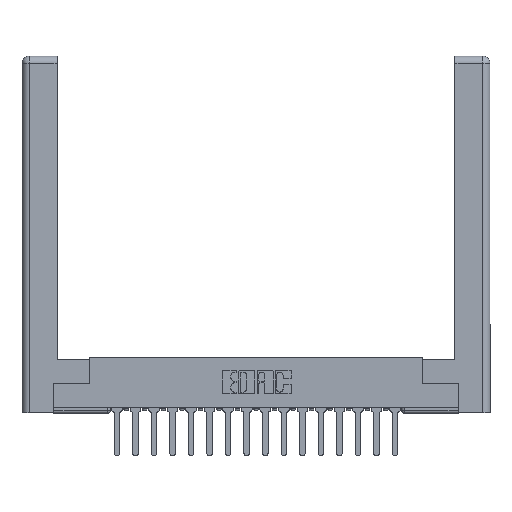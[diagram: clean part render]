
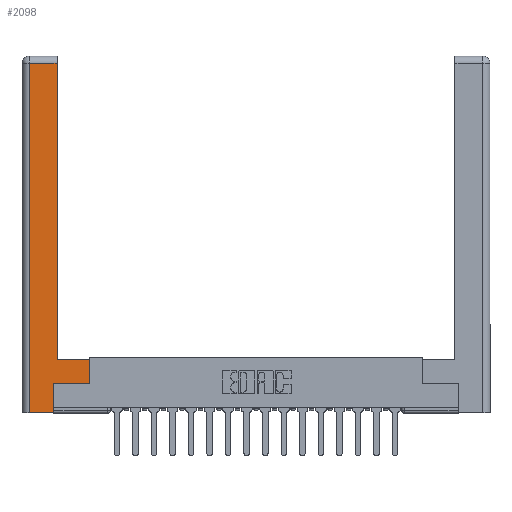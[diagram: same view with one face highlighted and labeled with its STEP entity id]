
A CAD part, top view. The second image highlights one B-rep face of the part: STEP entity #2098.
In plain terms, the highlighted planar face has unit normal (0, 0, 1).
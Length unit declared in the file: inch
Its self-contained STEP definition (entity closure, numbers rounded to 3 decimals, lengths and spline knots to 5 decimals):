
#366 = EDGE_CURVE ( 'NONE', #7946, #817, #15385, .T. ) ;
#458 = VECTOR ( 'NONE', #16230, 39.37008 ) ;
#817 = VERTEX_POINT ( 'NONE', #10457 ) ;
#1207 = AXIS2_PLACEMENT_3D ( 'NONE', #2498, #5435, #15996 ) ;
#1700 = VECTOR ( 'NONE', #7602, 39.37008 ) ;
#2098 = ADVANCED_FACE ( 'NONE', ( #2663 ), #11479, .F. ) ;
#2106 = EDGE_CURVE ( 'NONE', #19217, #8517, #2428, .T. ) ;
#2150 = VECTOR ( 'NONE', #5586, 39.37008 ) ;
#2428 = LINE ( 'NONE', #13015, #1700 ) ;
#2498 = CARTESIAN_POINT ( 'NONE',  ( 0., 0., 0. ) ) ;
#2663 = FACE_OUTER_BOUND ( 'NONE', #18390, .T. ) ;
#2796 = CARTESIAN_POINT ( 'NONE',  ( 0.295, 2.94, 0. ) ) ;
#3045 = LINE ( 'NONE', #8609, #458 ) ;
#3230 = EDGE_CURVE ( 'NONE', #817, #16304, #4022, .T. ) ;
#3514 = CARTESIAN_POINT ( 'NONE',  ( 0.265, 0.245, 0. ) ) ;
#3816 = VECTOR ( 'NONE', #17470, 39.37008 ) ;
#4022 = LINE ( 'NONE', #6672, #7511 ) ;
#4775 = ORIENTED_EDGE ( 'NONE', *, *, #3230, .T. ) ;
#5203 = CARTESIAN_POINT ( 'NONE',  ( 0.0615, 2.94, 0. ) ) ;
#5331 = EDGE_CURVE ( 'NONE', #12104, #14140, #7439, .T. ) ;
#5435 = DIRECTION ( 'NONE',  ( 0., 0., -1. ) ) ;
#5586 = DIRECTION ( 'NONE',  ( 1., 0., 0. ) ) ;
#6149 = LINE ( 'NONE', #13487, #2150 ) ;
#6268 = ORIENTED_EDGE ( 'NONE', *, *, #15713, .T. ) ;
#6672 = CARTESIAN_POINT ( 'NONE',  ( 0.295, 3., 0. ) ) ;
#7439 = LINE ( 'NONE', #7695, #16212 ) ;
#7511 = VECTOR ( 'NONE', #11032, 39.37008 ) ;
#7602 = DIRECTION ( 'NONE',  ( 0., -1., 0. ) ) ;
#7695 = CARTESIAN_POINT ( 'NONE',  ( 0.565, 0.245, 0. ) ) ;
#7751 = DIRECTION ( 'NONE',  ( 1., 0., 0. ) ) ;
#7946 = VERTEX_POINT ( 'NONE', #19038 ) ;
#8409 = CARTESIAN_POINT ( 'NONE',  ( 0.565, 0.245, 0. ) ) ;
#8517 = VERTEX_POINT ( 'NONE', #13154 ) ;
#8609 = CARTESIAN_POINT ( 'NONE',  ( 0.565, 0.45, 0. ) ) ;
#9453 = ORIENTED_EDGE ( 'NONE', *, *, #366, .T. ) ;
#9555 = DIRECTION ( 'NONE',  ( -1., 0., 0. ) ) ;
#9669 = VECTOR ( 'NONE', #9555, 39.37008 ) ;
#9711 = EDGE_CURVE ( 'NONE', #8517, #17462, #6149, .T. ) ;
#10340 = VECTOR ( 'NONE', #10469, 39.37008 ) ;
#10457 = CARTESIAN_POINT ( 'NONE',  ( 0.295, 0.45, 0. ) ) ;
#10469 = DIRECTION ( 'NONE',  ( -1., 0., 0. ) ) ;
#11032 = DIRECTION ( 'NONE',  ( 0., 1., 0. ) ) ;
#11479 = PLANE ( 'NONE',  #1207 ) ;
#12104 = VERTEX_POINT ( 'NONE', #3514 ) ;
#12984 = CARTESIAN_POINT ( 'NONE',  ( 0.265, 0.245, 0. ) ) ;
#13015 = CARTESIAN_POINT ( 'NONE',  ( 0.0615, 0., 0. ) ) ;
#13080 = ORIENTED_EDGE ( 'NONE', *, *, #16187, .T. ) ;
#13154 = CARTESIAN_POINT ( 'NONE',  ( 0.0615, 0., 0. ) ) ;
#13487 = CARTESIAN_POINT ( 'NONE',  ( 0.265, 0., 0. ) ) ;
#13966 = EDGE_CURVE ( 'NONE', #17462, #12104, #16313, .T. ) ;
#14011 = CARTESIAN_POINT ( 'NONE',  ( 0.295, 0.45, 0. ) ) ;
#14140 = VERTEX_POINT ( 'NONE', #8409 ) ;
#15305 = ORIENTED_EDGE ( 'NONE', *, *, #9711, .T. ) ;
#15379 = ORIENTED_EDGE ( 'NONE', *, *, #13966, .T. ) ;
#15385 = LINE ( 'NONE', #14011, #9669 ) ;
#15413 = ORIENTED_EDGE ( 'NONE', *, *, #2106, .T. ) ;
#15713 = EDGE_CURVE ( 'NONE', #16304, #19217, #16276, .T. ) ;
#15996 = DIRECTION ( 'NONE',  ( -1., 0., 0. ) ) ;
#16187 = EDGE_CURVE ( 'NONE', #14140, #7946, #3045, .T. ) ;
#16212 = VECTOR ( 'NONE', #7751, 39.37008 ) ;
#16230 = DIRECTION ( 'NONE',  ( 0., 1., 0. ) ) ;
#16276 = LINE ( 'NONE', #18016, #10340 ) ;
#16304 = VERTEX_POINT ( 'NONE', #2796 ) ;
#16313 = LINE ( 'NONE', #12984, #3816 ) ;
#17462 = VERTEX_POINT ( 'NONE', #17751 ) ;
#17470 = DIRECTION ( 'NONE',  ( 0., 1., 0. ) ) ;
#17751 = CARTESIAN_POINT ( 'NONE',  ( 0.265, 0., 0. ) ) ;
#18016 = CARTESIAN_POINT ( 'NONE',  ( 0.0615, 2.94, 0. ) ) ;
#18390 = EDGE_LOOP ( 'NONE', ( #4775, #6268, #15413, #15305, #15379, #18406, #13080, #9453 ) ) ;
#18406 = ORIENTED_EDGE ( 'NONE', *, *, #5331, .T. ) ;
#19038 = CARTESIAN_POINT ( 'NONE',  ( 0.565, 0.45, 0. ) ) ;
#19217 = VERTEX_POINT ( 'NONE', #5203 ) ;
